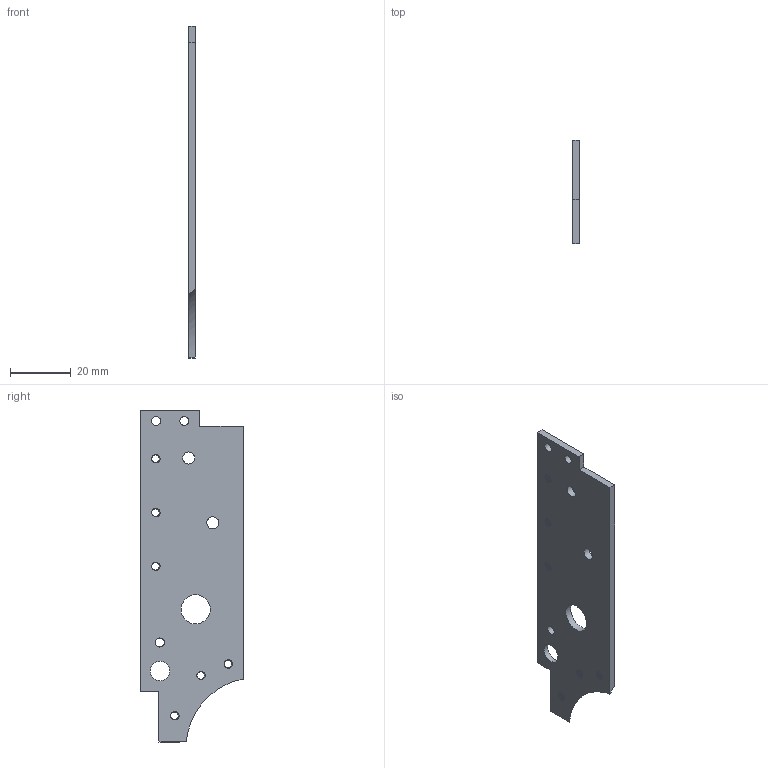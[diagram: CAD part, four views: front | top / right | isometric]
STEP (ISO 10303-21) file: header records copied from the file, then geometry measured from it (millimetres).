
FILE_DESCRIPTION(/* description */ (''),/* implementation_level */ '2;1');
FILE_NAME(/* name */ 'Rear SL Side Plate.step',/* time_stamp */ '2024-01-16T15:55:09-05:00',/* author */ (''),/* organization */ (''),/* preprocessor_version */ 'ST-DEVELOPER v20',/* originating_system */ 'Autodesk Translation Framework v12.14.0.127',/* authorisation */ '');
FILE_SCHEMA (('AUTOMOTIVE_DESIGN { 1 0 10303 214 3 1 1 }'));
Length unit declared in the file: inch
Products named in the file (1): Rear SL Side Plate
Bounding box: 2.29 x 33.91 x 109.73 mm (x, y, z)
Volume: 6898.7 mm3; surface area: 7165.8 mm2
Topology: 1 solids, 1 shells, 102 faces, 301 edges, 201 vertices
Faces by surface type: cylinder 75, plane 14, bspline 13
Full cylindrical faces by diameter (mm): 2.529 x6, 3 x3, 3.086 x6, 3.995 x2, 6.426 x1, 9.652 x1
Entity records: 7561 total; most frequent: CARTESIAN_POINT 5058, ORIENTED_EDGE 602, DIRECTION 362, EDGE_CURVE 301, VERTEX_POINT 201, B_SPLINE_CURVE_WITH_KNOTS 161, AXIS2_PLACEMENT_3D 132, EDGE_LOOP 128
